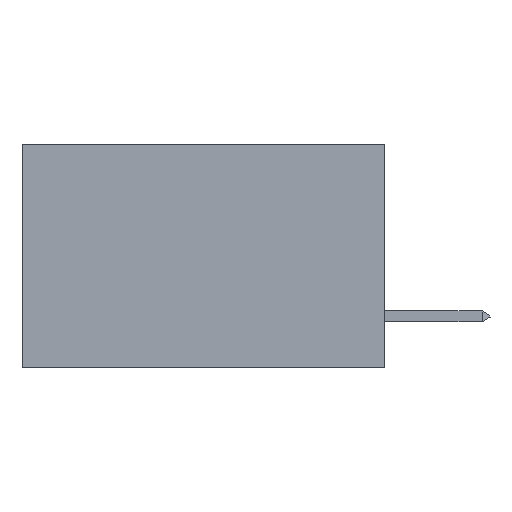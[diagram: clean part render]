
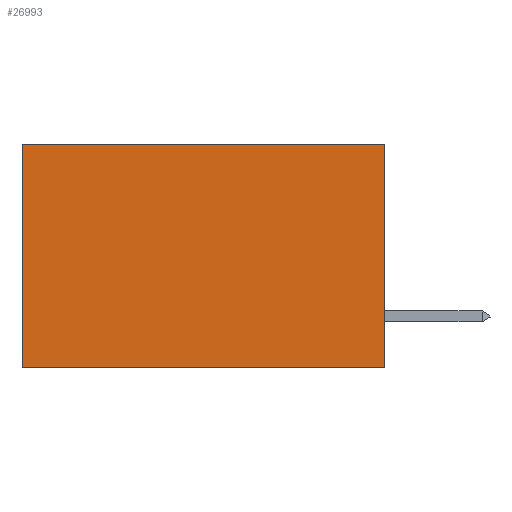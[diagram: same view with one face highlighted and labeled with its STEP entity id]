
A CAD part, left-side view. The second image highlights one B-rep face of the part: STEP entity #26993.
In plain terms, the highlighted planar face has unit normal (-1, 0, 0).
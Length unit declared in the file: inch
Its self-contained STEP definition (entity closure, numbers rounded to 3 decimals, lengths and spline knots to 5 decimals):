
#2520 = DIRECTION ( 'NONE',  ( 1., 0., 0. ) ) ;
#4751 = DIRECTION ( 'NONE',  ( 0., 0., -1. ) ) ;
#5395 = VECTOR ( 'NONE', #4751, 39.37008 ) ;
#6420 = CARTESIAN_POINT ( 'NONE',  ( 0.2875, 0., -0.37 ) ) ;
#7385 = CARTESIAN_POINT ( 'NONE',  ( 0.2875, 0.6, -0.37 ) ) ;
#8191 = CARTESIAN_POINT ( 'NONE',  ( 0.2875, 0., 0. ) ) ;
#8472 = EDGE_CURVE ( 'NONE', #25857, #19585, #32933, .T. ) ;
#9987 = AXIS2_PLACEMENT_3D ( 'NONE', #8191, #2520, #24571 ) ;
#11422 = LINE ( 'NONE', #27393, #5395 ) ;
#13347 = DIRECTION ( 'NONE',  ( 0., 1., 0. ) ) ;
#13611 = EDGE_CURVE ( 'NONE', #29460, #33765, #34728, .T. ) ;
#16116 = VECTOR ( 'NONE', #26253, 39.37008 ) ;
#17363 = VECTOR ( 'NONE', #13347, 39.37008 ) ;
#18788 = CARTESIAN_POINT ( 'NONE',  ( 0.2875, 0., -0.37 ) ) ;
#19585 = VERTEX_POINT ( 'NONE', #7385 ) ;
#21144 = ORIENTED_EDGE ( 'NONE', *, *, #8472, .F. ) ;
#21788 = PLANE ( 'NONE',  #9987 ) ;
#23080 = CARTESIAN_POINT ( 'NONE',  ( 0.2875, 0., 0. ) ) ;
#24571 = DIRECTION ( 'NONE',  ( 0., 0., -1. ) ) ;
#25178 = FACE_OUTER_BOUND ( 'NONE', #26357, .T. ) ;
#25857 = VERTEX_POINT ( 'NONE', #6420 ) ;
#26231 = DIRECTION ( 'NONE',  ( 0., 1., 0. ) ) ;
#26253 = DIRECTION ( 'NONE',  ( 0., 0., -1. ) ) ;
#26357 = EDGE_LOOP ( 'NONE', ( #34627, #21144, #26714, #26572 ) ) ;
#26572 = ORIENTED_EDGE ( 'NONE', *, *, #13611, .T. ) ;
#26710 = EDGE_CURVE ( 'NONE', #33765, #19585, #33777, .T. ) ;
#26714 = ORIENTED_EDGE ( 'NONE', *, *, #28740, .F. ) ;
#26993 = ADVANCED_FACE ( 'NONE', ( #25178 ), #21788, .F. ) ;
#27393 = CARTESIAN_POINT ( 'NONE',  ( 0.2875, 0., 0. ) ) ;
#28381 = CARTESIAN_POINT ( 'NONE',  ( 0.2875, 0., 0. ) ) ;
#28740 = EDGE_CURVE ( 'NONE', #29460, #25857, #11422, .T. ) ;
#29460 = VERTEX_POINT ( 'NONE', #28381 ) ;
#31005 = CARTESIAN_POINT ( 'NONE',  ( 0.2875, 0.6, 0. ) ) ;
#32933 = LINE ( 'NONE', #18788, #17363 ) ;
#33765 = VERTEX_POINT ( 'NONE', #31005 ) ;
#33777 = LINE ( 'NONE', #34617, #16116 ) ;
#34289 = VECTOR ( 'NONE', #26231, 39.37008 ) ;
#34617 = CARTESIAN_POINT ( 'NONE',  ( 0.2875, 0.6, 0. ) ) ;
#34627 = ORIENTED_EDGE ( 'NONE', *, *, #26710, .T. ) ;
#34728 = LINE ( 'NONE', #23080, #34289 ) ;
